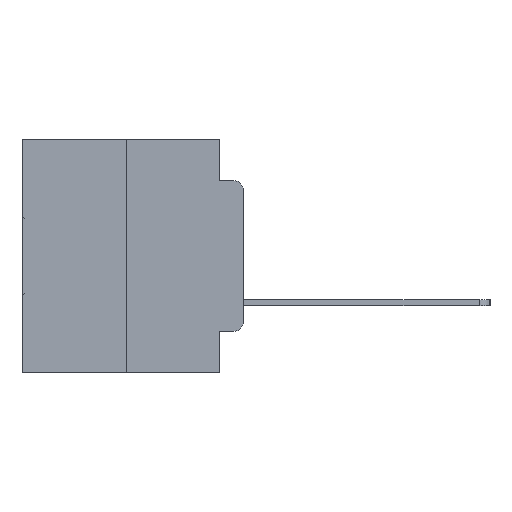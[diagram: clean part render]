
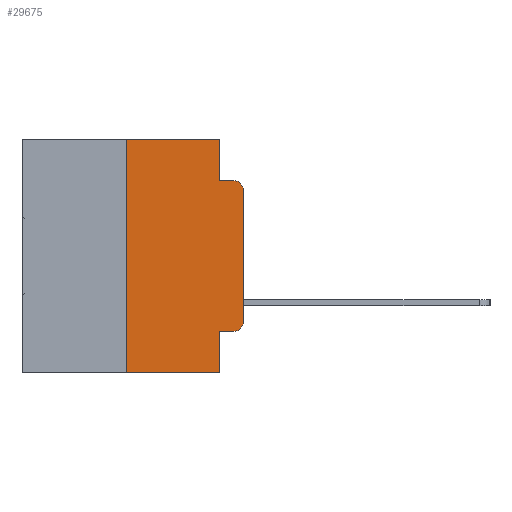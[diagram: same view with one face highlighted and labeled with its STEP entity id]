
A CAD part, left-side view. The second image highlights one B-rep face of the part: STEP entity #29675.
In plain terms, the highlighted planar face has unit normal (-1, 0, 0).
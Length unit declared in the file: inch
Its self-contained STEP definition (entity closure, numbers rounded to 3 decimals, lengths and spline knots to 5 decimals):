
#351 = CARTESIAN_POINT ( 'NONE',  ( 0., 0.25, 0. ) ) ;
#453 = VECTOR ( 'NONE', #763, 39.37008 ) ;
#763 = DIRECTION ( 'NONE',  ( 0., 0., 1. ) ) ;
#1177 = LINE ( 'NONE', #18037, #7016 ) ;
#1550 = ORIENTED_EDGE ( 'NONE', *, *, #6106, .F. ) ;
#2505 = VECTOR ( 'NONE', #31769, 39.37008 ) ;
#3121 = CARTESIAN_POINT ( 'NONE',  ( 0., 0.02, -0.0885 ) ) ;
#3287 = LINE ( 'NONE', #9785, #2505 ) ;
#3355 = EDGE_CURVE ( 'NONE', #15565, #24272, #18208, .T. ) ;
#4201 = CARTESIAN_POINT ( 'NONE',  ( 0., 0.051, -0.4115 ) ) ;
#4429 = DIRECTION ( 'NONE',  ( 1., 0., 0. ) ) ;
#5168 = VERTEX_POINT ( 'NONE', #4201 ) ;
#6106 = EDGE_CURVE ( 'NONE', #9252, #7346, #16548, .T. ) ;
#6350 = DIRECTION ( 'NONE',  ( 0., -1., 0. ) ) ;
#6689 = ORIENTED_EDGE ( 'NONE', *, *, #3355, .T. ) ;
#7016 = VECTOR ( 'NONE', #15573, 39.37008 ) ;
#7073 = CARTESIAN_POINT ( 'NONE',  ( 0., 0.051, -0.0885 ) ) ;
#7108 = LINE ( 'NONE', #21061, #13621 ) ;
#7346 = VERTEX_POINT ( 'NONE', #3121 ) ;
#7390 = DIRECTION ( 'NONE',  ( -1., 0., 0. ) ) ;
#8175 = CARTESIAN_POINT ( 'NONE',  ( 0., 0., 0. ) ) ;
#8397 = EDGE_CURVE ( 'NONE', #5168, #15565, #3287, .T. ) ;
#8471 = FACE_OUTER_BOUND ( 'NONE', #15546, .T. ) ;
#8927 = CARTESIAN_POINT ( 'NONE',  ( 0., 0.051, -0.5 ) ) ;
#9092 = VECTOR ( 'NONE', #18464, 39.37008 ) ;
#9252 = VERTEX_POINT ( 'NONE', #7073 ) ;
#9785 = CARTESIAN_POINT ( 'NONE',  ( 0., 0.051, -0.4115 ) ) ;
#12523 = AXIS2_PLACEMENT_3D ( 'NONE', #13045, #30142, #15494 ) ;
#12613 = VERTEX_POINT ( 'NONE', #8927 ) ;
#13045 = CARTESIAN_POINT ( 'NONE',  ( 0., 0.02, -0.3915 ) ) ;
#13553 = ORIENTED_EDGE ( 'NONE', *, *, #23840, .T. ) ;
#13621 = VECTOR ( 'NONE', #6350, 39.37008 ) ;
#14807 = VERTEX_POINT ( 'NONE', #20171 ) ;
#14943 = EDGE_CURVE ( 'NONE', #5168, #12613, #1177, .T. ) ;
#15044 = CIRCLE ( 'NONE', #16704, 0.02 ) ;
#15083 = ORIENTED_EDGE ( 'NONE', *, *, #14943, .F. ) ;
#15494 = DIRECTION ( 'NONE',  ( 0., 0., -1. ) ) ;
#15546 = EDGE_LOOP ( 'NONE', ( #27318, #28842, #1550, #16222, #22772, #17741, #13553, #15083, #16616, #6689 ) ) ;
#15565 = VERTEX_POINT ( 'NONE', #27874 ) ;
#15573 = DIRECTION ( 'NONE',  ( 0., 0., -1. ) ) ;
#15980 = EDGE_CURVE ( 'NONE', #23247, #7346, #15044, .T. ) ;
#16222 = ORIENTED_EDGE ( 'NONE', *, *, #31292, .F. ) ;
#16367 = LINE ( 'NONE', #30634, #9092 ) ;
#16548 = LINE ( 'NONE', #22931, #28804 ) ;
#16616 = ORIENTED_EDGE ( 'NONE', *, *, #8397, .T. ) ;
#16704 = AXIS2_PLACEMENT_3D ( 'NONE', #22081, #7390, #24537 ) ;
#17741 = ORIENTED_EDGE ( 'NONE', *, *, #23209, .F. ) ;
#18002 = VECTOR ( 'NONE', #26042, 39.37008 ) ;
#18037 = CARTESIAN_POINT ( 'NONE',  ( 0., 0.051, 0. ) ) ;
#18208 = CIRCLE ( 'NONE', #12523, 0.02 ) ;
#18464 = DIRECTION ( 'NONE',  ( 0., 0., -1. ) ) ;
#19175 = PLANE ( 'NONE',  #25514 ) ;
#19347 = EDGE_CURVE ( 'NONE', #14807, #21341, #7108, .T. ) ;
#20121 = LINE ( 'NONE', #8175, #453 ) ;
#20171 = CARTESIAN_POINT ( 'NONE',  ( 0., 0.25, 0. ) ) ;
#20188 = DIRECTION ( 'NONE',  ( 0., 0., 1. ) ) ;
#21061 = CARTESIAN_POINT ( 'NONE',  ( 0., 0.473, 0. ) ) ;
#21341 = VERTEX_POINT ( 'NONE', #22560 ) ;
#21674 = DIRECTION ( 'NONE',  ( 0., 0., -1. ) ) ;
#22081 = CARTESIAN_POINT ( 'NONE',  ( 0., 0.02, -0.1085 ) ) ;
#22560 = CARTESIAN_POINT ( 'NONE',  ( 0., 0.051, 0. ) ) ;
#22772 = ORIENTED_EDGE ( 'NONE', *, *, #19347, .F. ) ;
#22798 = CARTESIAN_POINT ( 'NONE',  ( 0., 0., -0.3915 ) ) ;
#22931 = CARTESIAN_POINT ( 'NONE',  ( 0., 0.051, -0.0885 ) ) ;
#23209 = EDGE_CURVE ( 'NONE', #30840, #14807, #29909, .T. ) ;
#23247 = VERTEX_POINT ( 'NONE', #27576 ) ;
#23789 = LINE ( 'NONE', #28370, #18002 ) ;
#23840 = EDGE_CURVE ( 'NONE', #30840, #12613, #23789, .T. ) ;
#24208 = VECTOR ( 'NONE', #20188, 39.37008 ) ;
#24272 = VERTEX_POINT ( 'NONE', #22798 ) ;
#24537 = DIRECTION ( 'NONE',  ( 0., 0., -1. ) ) ;
#25514 = AXIS2_PLACEMENT_3D ( 'NONE', #26497, #4429, #21674 ) ;
#26042 = DIRECTION ( 'NONE',  ( 0., -1., 0. ) ) ;
#26497 = CARTESIAN_POINT ( 'NONE',  ( 0., 0.473, 0. ) ) ;
#27318 = ORIENTED_EDGE ( 'NONE', *, *, #27479, .T. ) ;
#27479 = EDGE_CURVE ( 'NONE', #24272, #23247, #20121, .T. ) ;
#27576 = CARTESIAN_POINT ( 'NONE',  ( 0., 0., -0.1085 ) ) ;
#27828 = DIRECTION ( 'NONE',  ( 0., -1., 0. ) ) ;
#27874 = CARTESIAN_POINT ( 'NONE',  ( 0., 0.02, -0.4115 ) ) ;
#28370 = CARTESIAN_POINT ( 'NONE',  ( 0., 0.473, -0.5 ) ) ;
#28804 = VECTOR ( 'NONE', #27828, 39.37008 ) ;
#28842 = ORIENTED_EDGE ( 'NONE', *, *, #15980, .T. ) ;
#28861 = CARTESIAN_POINT ( 'NONE',  ( 0., 0.25, -0.5 ) ) ;
#29675 = ADVANCED_FACE ( 'NONE', ( #8471 ), #19175, .F. ) ;
#29909 = LINE ( 'NONE', #351, #24208 ) ;
#30142 = DIRECTION ( 'NONE',  ( -1., 0., 0. ) ) ;
#30634 = CARTESIAN_POINT ( 'NONE',  ( 0., 0.051, 0. ) ) ;
#30840 = VERTEX_POINT ( 'NONE', #28861 ) ;
#31292 = EDGE_CURVE ( 'NONE', #21341, #9252, #16367, .T. ) ;
#31769 = DIRECTION ( 'NONE',  ( 0., -1., 0. ) ) ;
